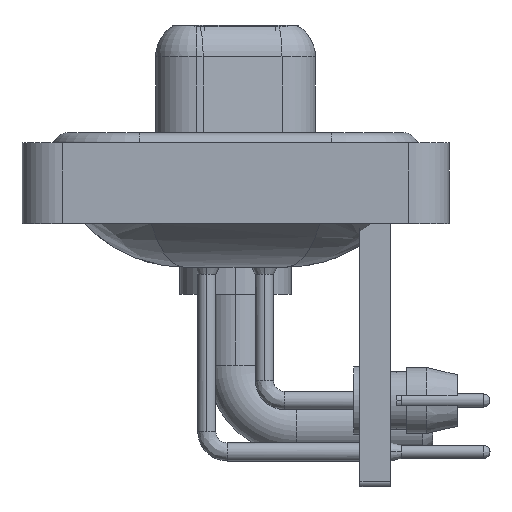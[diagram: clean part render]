
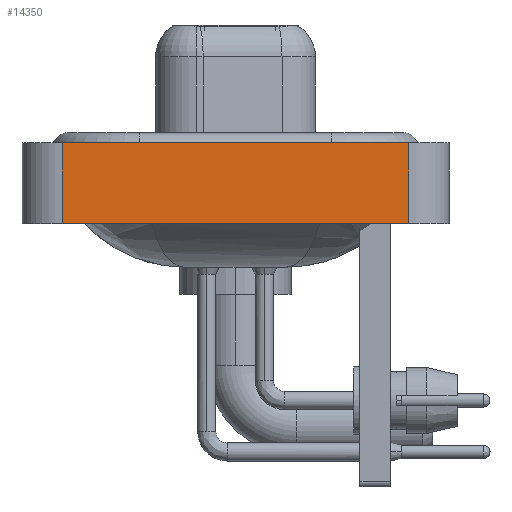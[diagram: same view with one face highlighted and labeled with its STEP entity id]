
A CAD part, left-side view. The second image highlights one B-rep face of the part: STEP entity #14350.
In plain terms, the highlighted planar face has unit normal (-1, 0, 0).
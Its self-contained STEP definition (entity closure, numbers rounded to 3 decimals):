
#1047 = CARTESIAN_POINT ( 'NONE',  ( -7.35, 8.55, -3.6 ) ) ;
#1154 = VECTOR ( 'NONE', #24205, 1000. ) ;
#1549 = VECTOR ( 'NONE', #27010, 1000. ) ;
#2348 = CARTESIAN_POINT ( 'NONE',  ( -7.35, 8.55, -3.6 ) ) ;
#3774 = CARTESIAN_POINT ( 'NONE',  ( -7.35, -8.55, -3.6 ) ) ;
#4781 = VECTOR ( 'NONE', #24961, 1000. ) ;
#5078 = EDGE_CURVE ( 'NONE', #24398, #25135, #13112, .T. ) ;
#6095 = VERTEX_POINT ( 'NONE', #14123 ) ;
#6399 = FACE_OUTER_BOUND ( 'NONE', #28418, .T. ) ;
#7154 = CARTESIAN_POINT ( 'NONE',  ( -7.35, -8.55, -3.6 ) ) ;
#9235 = ORIENTED_EDGE ( 'NONE', *, *, #12088, .F. ) ;
#9838 = EDGE_CURVE ( 'NONE', #25135, #6095, #27146, .T. ) ;
#12088 = EDGE_CURVE ( 'NONE', #24398, #14174, #18076, .T. ) ;
#12835 = AXIS2_PLACEMENT_3D ( 'NONE', #3774, #22159, #18029 ) ;
#13112 = LINE ( 'NONE', #28028, #1154 ) ;
#13920 = CARTESIAN_POINT ( 'NONE',  ( -7.35, -8.55, -3.6 ) ) ;
#14123 = CARTESIAN_POINT ( 'NONE',  ( -7.35, -8.55, 0.4 ) ) ;
#14174 = VERTEX_POINT ( 'NONE', #23479 ) ;
#14350 = ADVANCED_FACE ( 'NONE', ( #6399 ), #24184, .T. ) ;
#14739 = ORIENTED_EDGE ( 'NONE', *, *, #5078, .T. ) ;
#15332 = CARTESIAN_POINT ( 'NONE',  ( -7.35, -8.55, 0.4 ) ) ;
#15546 = ORIENTED_EDGE ( 'NONE', *, *, #9838, .T. ) ;
#17739 = EDGE_CURVE ( 'NONE', #14174, #6095, #19697, .T. ) ;
#18029 = DIRECTION ( 'NONE',  ( 0., 0., 1. ) ) ;
#18076 = LINE ( 'NONE', #2348, #1549 ) ;
#18618 = VECTOR ( 'NONE', #26295, 1000. ) ;
#19697 = LINE ( 'NONE', #15332, #18618 ) ;
#22159 = DIRECTION ( 'NONE',  ( -1., 0., 0. ) ) ;
#23479 = CARTESIAN_POINT ( 'NONE',  ( -7.35, 8.55, 0.4 ) ) ;
#24184 = PLANE ( 'NONE',  #12835 ) ;
#24205 = DIRECTION ( 'NONE',  ( 0., -1., 0. ) ) ;
#24398 = VERTEX_POINT ( 'NONE', #1047 ) ;
#24833 = ORIENTED_EDGE ( 'NONE', *, *, #17739, .F. ) ;
#24961 = DIRECTION ( 'NONE',  ( 0., 0., 1. ) ) ;
#25135 = VERTEX_POINT ( 'NONE', #13920 ) ;
#26295 = DIRECTION ( 'NONE',  ( 0., -1., 0. ) ) ;
#27010 = DIRECTION ( 'NONE',  ( 0., 0., 1. ) ) ;
#27146 = LINE ( 'NONE', #7154, #4781 ) ;
#28028 = CARTESIAN_POINT ( 'NONE',  ( -7.35, -8.55, -3.6 ) ) ;
#28418 = EDGE_LOOP ( 'NONE', ( #15546, #24833, #9235, #14739 ) ) ;
